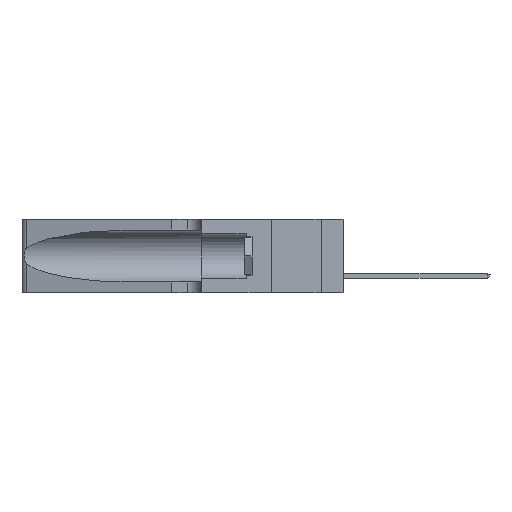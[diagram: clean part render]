
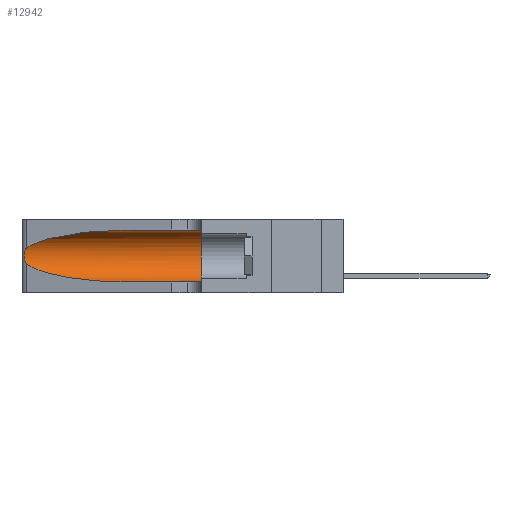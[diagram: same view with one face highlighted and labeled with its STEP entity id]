
A CAD part, left-side view. The second image highlights one B-rep face of the part: STEP entity #12942.
In plain terms, the highlighted cylindrical face has radius 3.308 mm (diameter 6.617 mm), a partial arc.
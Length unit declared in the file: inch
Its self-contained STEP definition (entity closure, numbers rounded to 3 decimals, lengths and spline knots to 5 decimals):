
#397 = DIRECTION ( 'NONE',  ( 0., -1., 0. ) ) ;
#537 = CARTESIAN_POINT ( 'NONE',  ( 0.25639, 1.23186, 0.15144 ) ) ;
#722 = CARTESIAN_POINT ( 'NONE',  ( 0.1305, 1.61858, 0.31525 ) ) ;
#1795 = B_SPLINE_CURVE_WITH_KNOTS ( 'NONE', 3,
 ( #35739, #42825, #15237, #21817, #39758, #43297, #25393, #14632, #25240, #32828, #11698, #537, #43456, #22283 ),
 .UNSPECIFIED., .F., .F.,
 ( 4, 2, 2, 2, 2, 2, 4 ),
 ( 0., 0.00027, 0.00053, 0.00107, 0.0016, 0.00187, 0.00214 ),
 .UNSPECIFIED. ) ;
#2642 = VERTEX_POINT ( 'NONE', #21373 ) ;
#3923 = VERTEX_POINT ( 'NONE', #20341 ) ;
#5915 = CIRCLE ( 'NONE', #23304, 0.13025 ) ;
#6685 = CARTESIAN_POINT ( 'NONE',  ( 0.1305, 0.35, 0.185 ) ) ;
#7763 = ORIENTED_EDGE ( 'NONE', *, *, #24421, .F. ) ;
#9534 = CARTESIAN_POINT ( 'NONE',  ( 0.18966, 0.96281, 0.31525 ) ) ;
#9988 = CARTESIAN_POINT ( 'NONE',  ( 0.25487, 1.22718, 0.22369 ) ) ;
#10864 = EDGE_CURVE ( 'NONE', #36277, #40734, #16254, .T. ) ;
#11488 = DIRECTION ( 'NONE',  ( 0., 0., -1. ) ) ;
#11698 = CARTESIAN_POINT ( 'NONE',  ( 0.25789, 1.23486, 0.15765 ) ) ;
#12942 = ADVANCED_FACE ( 'NONE', ( #31406 ), #13750, .F. ) ;
#13341 = DIRECTION ( 'NONE',  ( 0., 0., 1. ) ) ;
#13750 = CYLINDRICAL_SURFACE ( 'NONE', #19906, 0.13025 ) ;
#14388 = EDGE_CURVE ( 'NONE', #14770, #36277, #1795, .T. ) ;
#14399 = CARTESIAN_POINT ( 'NONE',  ( 0.25487, 1.22718, 0.14631 ) ) ;
#14632 = CARTESIAN_POINT ( 'NONE',  ( 0.26075, 1.23896, 0.178 ) ) ;
#14770 = VERTEX_POINT ( 'NONE', #39239 ) ;
#15237 = CARTESIAN_POINT ( 'NONE',  ( 0.25639, 1.23184, 0.21858 ) ) ;
#15725 = ORIENTED_EDGE ( 'NONE', *, *, #14388, .T. ) ;
#16240 = LINE ( 'NONE', #722, #34474 ) ;
#16254 =( BOUNDED_CURVE ( )  B_SPLINE_CURVE ( 3, ( #24259, #27364, #16876, #20693 ),
 .UNSPECIFIED., .F., .F. ) 
 B_SPLINE_CURVE_WITH_KNOTS ( ( 4, 4 ),
 ( 3.44316, 4.71239 ),
 .UNSPECIFIED. ) 
 CURVE ( )  GEOMETRIC_REPRESENTATION_ITEM ( )  RATIONAL_B_SPLINE_CURVE ( ( 1., 0.87, 0.87, 1. ) ) 
 REPRESENTATION_ITEM ( '' )  );
#16876 = CARTESIAN_POINT ( 'NONE',  ( 0.18966, 0.96281, 0.05475 ) ) ;
#19906 = AXIS2_PLACEMENT_3D ( 'NONE', #43082, #21914, #11488 ) ;
#20341 = CARTESIAN_POINT ( 'NONE',  ( 0.1305, 0.35, 0.05475 ) ) ;
#20693 = CARTESIAN_POINT ( 'NONE',  ( 0.1305, 0.72297, 0.05475 ) ) ;
#21373 = CARTESIAN_POINT ( 'NONE',  ( 0.1305, 0.35, 0.31525 ) ) ;
#21817 = CARTESIAN_POINT ( 'NONE',  ( 0.25787, 1.23484, 0.2124 ) ) ;
#21914 = DIRECTION ( 'NONE',  ( 0., -1., 0. ) ) ;
#22283 = CARTESIAN_POINT ( 'NONE',  ( 0.25487, 1.22718, 0.14631 ) ) ;
#23304 = AXIS2_PLACEMENT_3D ( 'NONE', #6685, #24248, #13341 ) ;
#23523 = CARTESIAN_POINT ( 'NONE',  ( 0.2373, 1.15595, 0.28018 ) ) ;
#24248 = DIRECTION ( 'NONE',  ( 0., 1., 0. ) ) ;
#24259 = CARTESIAN_POINT ( 'NONE',  ( 0.25487, 1.22718, 0.14631 ) ) ;
#24421 = EDGE_CURVE ( 'NONE', #2642, #3923, #5915, .T. ) ;
#25148 = VERTEX_POINT ( 'NONE', #33979 ) ;
#25240 = CARTESIAN_POINT ( 'NONE',  ( 0.26017, 1.23833, 0.17102 ) ) ;
#25393 = CARTESIAN_POINT ( 'NONE',  ( 0.26075, 1.23896, 0.19203 ) ) ;
#26580 = ORIENTED_EDGE ( 'NONE', *, *, #31561, .T. ) ;
#26878 = EDGE_LOOP ( 'NONE', ( #37590, #15725, #33169, #26580, #7763, #27803 ) ) ;
#26929 = CARTESIAN_POINT ( 'NONE',  ( 0.1305, 0.72297, 0.31525 ) ) ;
#27364 = CARTESIAN_POINT ( 'NONE',  ( 0.2373, 1.15595, 0.08982 ) ) ;
#27594 = VECTOR ( 'NONE', #397, 39.37008 ) ;
#27803 = ORIENTED_EDGE ( 'NONE', *, *, #29300, .F. ) ;
#29212 =( BOUNDED_CURVE ( )  B_SPLINE_CURVE ( 3, ( #26929, #9534, #23523, #9988 ),
 .UNSPECIFIED., .F., .F. ) 
 B_SPLINE_CURVE_WITH_KNOTS ( ( 4, 4 ),
 ( 1.5708, 2.84003 ),
 .UNSPECIFIED. ) 
 CURVE ( )  GEOMETRIC_REPRESENTATION_ITEM ( )  RATIONAL_B_SPLINE_CURVE ( ( 1., 0.87, 0.87, 1. ) ) 
 REPRESENTATION_ITEM ( '' )  );
#29300 = EDGE_CURVE ( 'NONE', #25148, #2642, #16240, .T. ) ;
#31406 = FACE_OUTER_BOUND ( 'NONE', #26878, .T. ) ;
#31561 = EDGE_CURVE ( 'NONE', #40734, #3923, #33139, .T. ) ;
#32531 = CARTESIAN_POINT ( 'NONE',  ( 0.1305, 1.61858, 0.05475 ) ) ;
#32828 = CARTESIAN_POINT ( 'NONE',  ( 0.25856, 1.23593, 0.16098 ) ) ;
#33139 = LINE ( 'NONE', #32531, #27594 ) ;
#33169 = ORIENTED_EDGE ( 'NONE', *, *, #10864, .T. ) ;
#33667 = EDGE_CURVE ( 'NONE', #25148, #14770, #29212, .T. ) ;
#33979 = CARTESIAN_POINT ( 'NONE',  ( 0.1305, 0.72297, 0.31525 ) ) ;
#34474 = VECTOR ( 'NONE', #44120, 39.37008 ) ;
#35739 = CARTESIAN_POINT ( 'NONE',  ( 0.25487, 1.22718, 0.22369 ) ) ;
#36277 = VERTEX_POINT ( 'NONE', #14399 ) ;
#37590 = ORIENTED_EDGE ( 'NONE', *, *, #33667, .T. ) ;
#39239 = CARTESIAN_POINT ( 'NONE',  ( 0.25487, 1.22718, 0.22369 ) ) ;
#39758 = CARTESIAN_POINT ( 'NONE',  ( 0.25854, 1.2359, 0.20912 ) ) ;
#40734 = VERTEX_POINT ( 'NONE', #43303 ) ;
#42825 = CARTESIAN_POINT ( 'NONE',  ( 0.25555, 1.22994, 0.2215 ) ) ;
#43082 = CARTESIAN_POINT ( 'NONE',  ( 0.1305, 1.61858, 0.185 ) ) ;
#43297 = CARTESIAN_POINT ( 'NONE',  ( 0.26018, 1.23835, 0.19895 ) ) ;
#43303 = CARTESIAN_POINT ( 'NONE',  ( 0.1305, 0.72297, 0.05475 ) ) ;
#43456 = CARTESIAN_POINT ( 'NONE',  ( 0.25555, 1.22993, 0.14849 ) ) ;
#44120 = DIRECTION ( 'NONE',  ( 0., -1., 0. ) ) ;
